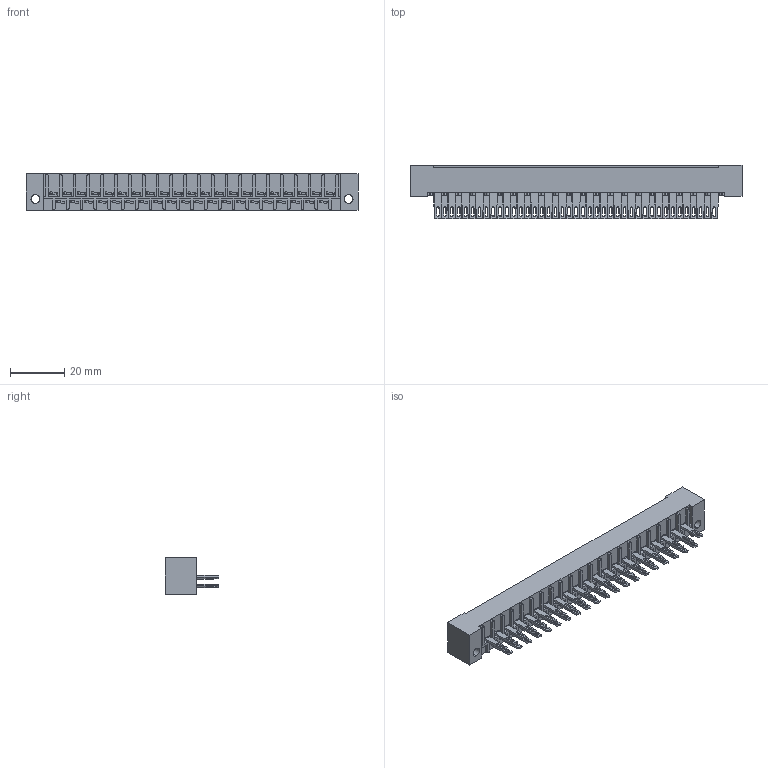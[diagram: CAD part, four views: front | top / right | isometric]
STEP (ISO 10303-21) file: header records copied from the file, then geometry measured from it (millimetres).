
FILE_DESCRIPTION (( 'STEP AP203' ), '1' );
FILE_NAME ('408-047-500-112.STEP', '2019-11-04T19:39:20', ( '' ), ( '' ), 'SwSTEP 2.0', 'SolidWorks 2016', '' );
FILE_SCHEMA (( 'CONFIG_CONTROL_DESIGN' ));
Length unit declared in the file: inch
Products named in the file (3): 408 Part_041 - 1; 408-290-001_408-290-100; 408-047-500-112
Assembly tree (42 placements, depth 2):
  408-047-500-112
    408 Part_041 - 1
    408-290-001_408-290-100  x41
Bounding box: 122.07 x 19.79 x 13.49 mm (x, y, z)
Volume: 14317.6 mm3; surface area: 18265 mm2
Topology: 42 solids, 42 shells, 2381 faces, 6559 edges, 4262 vertices
Faces by surface type: plane 1717, cylinder 500, bspline 164
Entity records: 27572 total; most frequent: CARTESIAN_POINT 4743, ORIENTED_EDGE 4638, DIRECTION 4155, EDGE_CURVE 2319, LINE 2119, VECTOR 2119, VERTEX_POINT 1542, AXIS2_PLACEMENT_3D 1018
